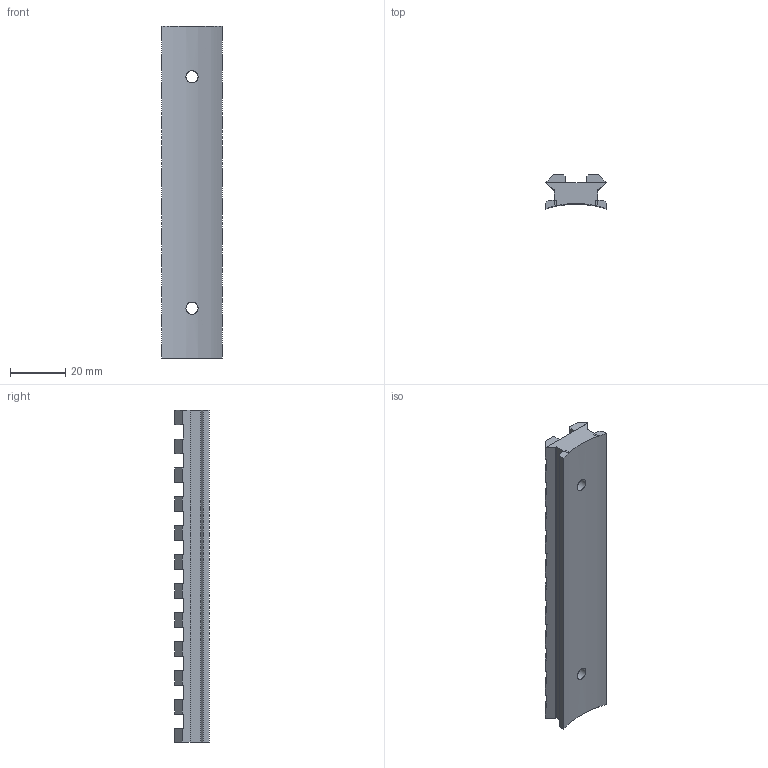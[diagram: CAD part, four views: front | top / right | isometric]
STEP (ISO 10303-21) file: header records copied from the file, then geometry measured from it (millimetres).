
FILE_DESCRIPTION(('FreeCAD Model'),'2;1');
FILE_NAME('mp-1 sight rail.step' ,'2016-02-20T15:48:00',('Author'),(''), 'Open CASCADE STEP processor 6.8','FreeCAD','Unknown');
FILE_SCHEMA(('AUTOMOTIVE_DESIGN_CC2 { 1 2 10303 214 -1 1 5 4 }'));
Length unit declared in the file: millimetre
Products named in the file (1): Chamfer001
Bounding box: 22 x 12.38 x 120 mm (x, y, z)
Volume: 18951.9 mm3; surface area: 10359.9 mm2
Topology: 1 solids, 1 shells, 184 faces, 530 edges, 348 vertices
Faces by surface type: plane 177, cylinder 7
Full cylindrical faces by diameter (mm): 4.4 x2, 8.4 x2
Entity records: 13504 total; most frequent: CARTESIAN_POINT 2961, DIRECTION 1901, LINE 1480, VECTOR 1480, ORIENTED_EDGE 1064, PCURVE 1060, DEFINITIONAL_REPRESENTATION 1060, EDGE_CURVE 530
